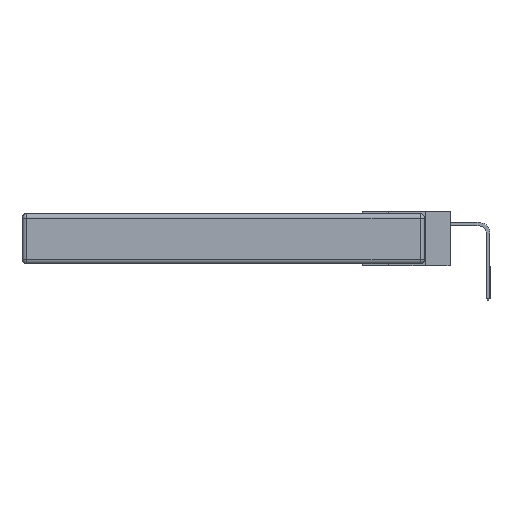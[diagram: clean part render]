
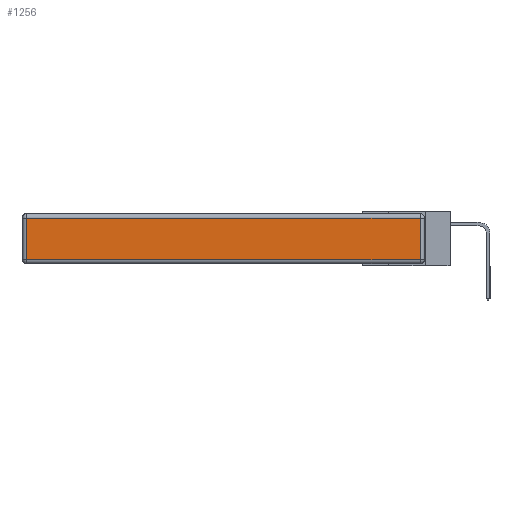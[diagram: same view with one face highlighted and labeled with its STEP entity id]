
A CAD part, left-side view. The second image highlights one B-rep face of the part: STEP entity #1256.
In plain terms, the highlighted planar face has unit normal (-1, 0, 0).
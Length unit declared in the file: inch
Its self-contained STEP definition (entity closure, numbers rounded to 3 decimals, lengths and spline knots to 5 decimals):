
#1256 = ADVANCED_FACE ( 'NONE', ( #28532 ), #10142, .T. ) ;
#1483 = DIRECTION ( 'NONE',  ( 0., 0., 1. ) ) ;
#1796 = VECTOR ( 'NONE', #1483, 39.37008 ) ;
#1897 = EDGE_CURVE ( 'NONE', #10008, #21983, #16141, .T. ) ;
#1985 = EDGE_LOOP ( 'NONE', ( #29579, #12046, #32403, #28103 ) ) ;
#3468 = AXIS2_PLACEMENT_3D ( 'NONE', #10027, #12592, #27978 ) ;
#4653 = CARTESIAN_POINT ( 'NONE',  ( 0., 2.75, -0.03 ) ) ;
#5199 = DIRECTION ( 'NONE',  ( 0., 0., -1. ) ) ;
#5523 = VECTOR ( 'NONE', #5199, 39.37008 ) ;
#7298 = EDGE_CURVE ( 'NONE', #8152, #10008, #31962, .T. ) ;
#7790 = VECTOR ( 'NONE', #17435, 39.37008 ) ;
#8152 = VERTEX_POINT ( 'NONE', #28589 ) ;
#8325 = VERTEX_POINT ( 'NONE', #22093 ) ;
#9966 = DIRECTION ( 'NONE',  ( 0., 1., 0. ) ) ;
#10008 = VERTEX_POINT ( 'NONE', #21507 ) ;
#10027 = CARTESIAN_POINT ( 'NONE',  ( 0., 0., -0.343 ) ) ;
#10142 = PLANE ( 'NONE',  #3468 ) ;
#11666 = EDGE_CURVE ( 'NONE', #21983, #8325, #17300, .T. ) ;
#11772 = EDGE_CURVE ( 'NONE', #8325, #8152, #14109, .T. ) ;
#12046 = ORIENTED_EDGE ( 'NONE', *, *, #11666, .T. ) ;
#12532 = CARTESIAN_POINT ( 'NONE',  ( 0., 2.72, -0.343 ) ) ;
#12592 = DIRECTION ( 'NONE',  ( -1., 0., 0. ) ) ;
#14109 = LINE ( 'NONE', #4653, #22489 ) ;
#16141 = LINE ( 'NONE', #31940, #7790 ) ;
#17300 = LINE ( 'NONE', #21653, #1796 ) ;
#17435 = DIRECTION ( 'NONE',  ( 0., -1., 0. ) ) ;
#21507 = CARTESIAN_POINT ( 'NONE',  ( 0., 2.72, -0.313 ) ) ;
#21653 = CARTESIAN_POINT ( 'NONE',  ( 0., 0.03, -0.343 ) ) ;
#21983 = VERTEX_POINT ( 'NONE', #21984 ) ;
#21984 = CARTESIAN_POINT ( 'NONE',  ( 0., 0.03, -0.313 ) ) ;
#22093 = CARTESIAN_POINT ( 'NONE',  ( 0., 0.03, -0.03 ) ) ;
#22489 = VECTOR ( 'NONE', #9966, 39.37008 ) ;
#27978 = DIRECTION ( 'NONE',  ( 0., 0., 1. ) ) ;
#28103 = ORIENTED_EDGE ( 'NONE', *, *, #7298, .T. ) ;
#28532 = FACE_OUTER_BOUND ( 'NONE', #1985, .T. ) ;
#28589 = CARTESIAN_POINT ( 'NONE',  ( 0., 2.72, -0.03 ) ) ;
#29579 = ORIENTED_EDGE ( 'NONE', *, *, #1897, .T. ) ;
#31940 = CARTESIAN_POINT ( 'NONE',  ( 0., 0., -0.313 ) ) ;
#31962 = LINE ( 'NONE', #12532, #5523 ) ;
#32403 = ORIENTED_EDGE ( 'NONE', *, *, #11772, .T. ) ;
